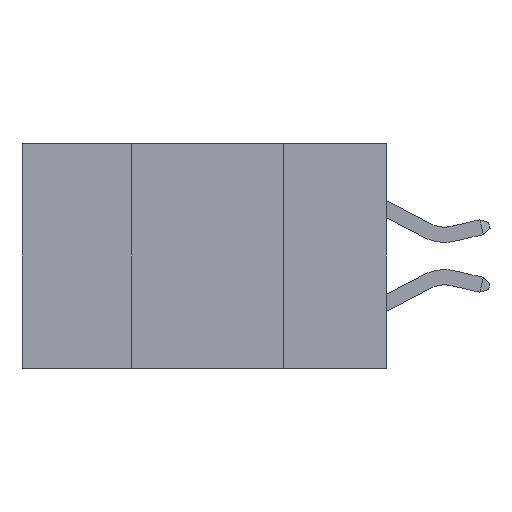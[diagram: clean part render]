
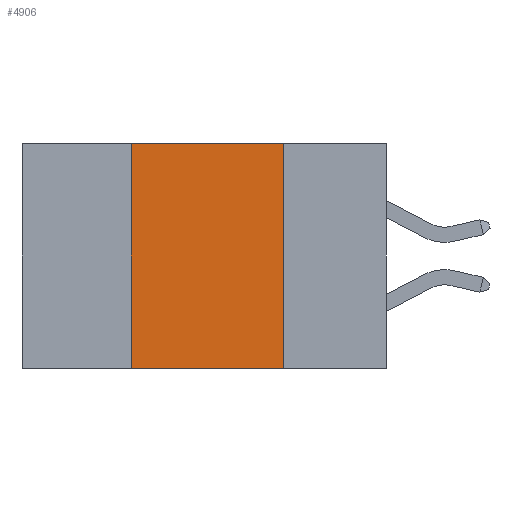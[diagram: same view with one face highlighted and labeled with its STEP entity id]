
A CAD part, left-side view. The second image highlights one B-rep face of the part: STEP entity #4906.
In plain terms, the highlighted planar face has unit normal (-1, 0, 0).
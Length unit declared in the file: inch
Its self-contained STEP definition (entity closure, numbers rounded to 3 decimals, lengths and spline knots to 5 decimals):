
#288 = CARTESIAN_POINT ( 'NONE',  ( 0., 0.42, -0.37 ) ) ;
#554 = LINE ( 'NONE', #14090, #17676 ) ;
#619 = DIRECTION ( 'NONE',  ( 0., -1., 0. ) ) ;
#806 = CARTESIAN_POINT ( 'NONE',  ( 0., 0.42, -0.37 ) ) ;
#1178 = ORIENTED_EDGE ( 'NONE', *, *, #6165, .F. ) ;
#1200 = CARTESIAN_POINT ( 'NONE',  ( 0., 0.17, 0. ) ) ;
#1587 = ORIENTED_EDGE ( 'NONE', *, *, #9196, .T. ) ;
#2210 = LINE ( 'NONE', #288, #17942 ) ;
#3019 = VERTEX_POINT ( 'NONE', #15446 ) ;
#3101 = PLANE ( 'NONE',  #10190 ) ;
#3700 = EDGE_CURVE ( 'NONE', #19690, #3019, #21742, .T. ) ;
#3971 = CARTESIAN_POINT ( 'NONE',  ( 0., 0.42, 0. ) ) ;
#4906 = ADVANCED_FACE ( 'NONE', ( #14945 ), #3101, .F. ) ;
#5940 = VECTOR ( 'NONE', #619, 39.37008 ) ;
#6165 = EDGE_CURVE ( 'NONE', #6605, #19690, #554, .T. ) ;
#6486 = DIRECTION ( 'NONE',  ( 0., 0., -1. ) ) ;
#6605 = VERTEX_POINT ( 'NONE', #3971 ) ;
#8811 = EDGE_LOOP ( 'NONE', ( #18460, #1178, #10852, #1587 ) ) ;
#9196 = EDGE_CURVE ( 'NONE', #11344, #3019, #21251, .T. ) ;
#9551 = DIRECTION ( 'NONE',  ( 0., 0., -1. ) ) ;
#10190 = AXIS2_PLACEMENT_3D ( 'NONE', #15056, #21943, #6486 ) ;
#10852 = ORIENTED_EDGE ( 'NONE', *, *, #19963, .F. ) ;
#11344 = VERTEX_POINT ( 'NONE', #806 ) ;
#11479 = CARTESIAN_POINT ( 'NONE',  ( 0., 0.17, -0.37 ) ) ;
#11883 = VECTOR ( 'NONE', #9551, 39.37008 ) ;
#14090 = CARTESIAN_POINT ( 'NONE',  ( 0., 0.6, 0. ) ) ;
#14945 = FACE_OUTER_BOUND ( 'NONE', #8811, .T. ) ;
#15056 = CARTESIAN_POINT ( 'NONE',  ( 0., 0.6, 0. ) ) ;
#15446 = CARTESIAN_POINT ( 'NONE',  ( 0., 0.17, -0.37 ) ) ;
#17639 = DIRECTION ( 'NONE',  ( 0., 0., 1. ) ) ;
#17676 = VECTOR ( 'NONE', #21301, 39.37008 ) ;
#17942 = VECTOR ( 'NONE', #17639, 39.37008 ) ;
#18460 = ORIENTED_EDGE ( 'NONE', *, *, #3700, .F. ) ;
#19690 = VERTEX_POINT ( 'NONE', #1200 ) ;
#19900 = CARTESIAN_POINT ( 'NONE',  ( 0., 0.6, -0.37 ) ) ;
#19963 = EDGE_CURVE ( 'NONE', #11344, #6605, #2210, .T. ) ;
#21251 = LINE ( 'NONE', #19900, #5940 ) ;
#21301 = DIRECTION ( 'NONE',  ( 0., -1., 0. ) ) ;
#21742 = LINE ( 'NONE', #11479, #11883 ) ;
#21943 = DIRECTION ( 'NONE',  ( 1., 0., 0. ) ) ;
